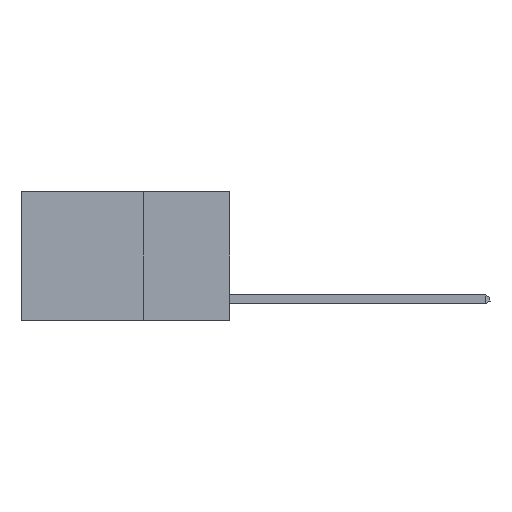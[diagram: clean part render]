
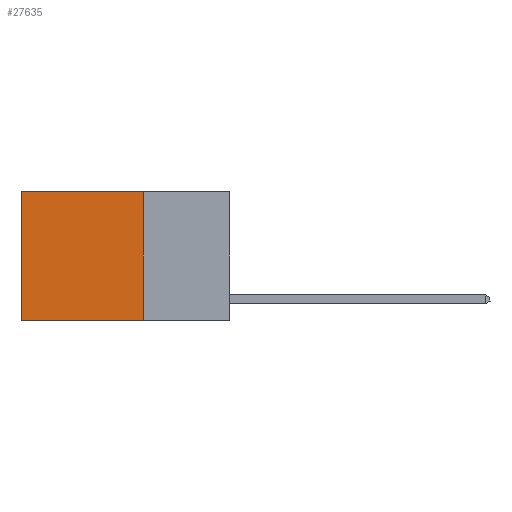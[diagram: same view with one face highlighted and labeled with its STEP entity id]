
A CAD part, left-side view. The second image highlights one B-rep face of the part: STEP entity #27635.
In plain terms, the highlighted planar face has unit normal (-1, 0, 0).
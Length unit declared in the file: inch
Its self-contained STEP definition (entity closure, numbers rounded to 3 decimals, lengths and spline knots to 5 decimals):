
#2119 = ORIENTED_EDGE ( 'NONE', *, *, #8490, .T. ) ;
#3707 = CARTESIAN_POINT ( 'NONE',  ( 0.2625, 0.25, -0.37 ) ) ;
#5511 = LINE ( 'NONE', #29322, #12261 ) ;
#5602 = AXIS2_PLACEMENT_3D ( 'NONE', #17072, #10039, #26756 ) ;
#6097 = LINE ( 'NONE', #23149, #17379 ) ;
#6677 = VERTEX_POINT ( 'NONE', #13374 ) ;
#8291 = LINE ( 'NONE', #10303, #20652 ) ;
#8490 = EDGE_CURVE ( 'NONE', #20368, #9967, #23485, .T. ) ;
#8872 = CARTESIAN_POINT ( 'NONE',  ( 0.2625, 0.6, 0. ) ) ;
#8935 = ORIENTED_EDGE ( 'NONE', *, *, #17023, .F. ) ;
#8991 = CARTESIAN_POINT ( 'NONE',  ( 0.2625, 0.6, 0. ) ) ;
#9967 = VERTEX_POINT ( 'NONE', #22264 ) ;
#10039 = DIRECTION ( 'NONE',  ( 1., 0., 0. ) ) ;
#10198 = DIRECTION ( 'NONE',  ( 0., 1., 0. ) ) ;
#10303 = CARTESIAN_POINT ( 'NONE',  ( 0.2625, 0.25, -0.37 ) ) ;
#11815 = VECTOR ( 'NONE', #28025, 39.37008 ) ;
#12261 = VECTOR ( 'NONE', #12357, 39.37008 ) ;
#12357 = DIRECTION ( 'NONE',  ( 0., 0., -1. ) ) ;
#13374 = CARTESIAN_POINT ( 'NONE',  ( 0.2625, 0.25, 0. ) ) ;
#13723 = ORIENTED_EDGE ( 'NONE', *, *, #22819, .T. ) ;
#16827 = EDGE_LOOP ( 'NONE', ( #2119, #8935, #21894, #13723 ) ) ;
#17023 = EDGE_CURVE ( 'NONE', #28780, #9967, #8291, .T. ) ;
#17072 = CARTESIAN_POINT ( 'NONE',  ( 0.2625, 0.25, 0. ) ) ;
#17379 = VECTOR ( 'NONE', #25351, 39.37008 ) ;
#20368 = VERTEX_POINT ( 'NONE', #8991 ) ;
#20652 = VECTOR ( 'NONE', #10198, 39.37008 ) ;
#21894 = ORIENTED_EDGE ( 'NONE', *, *, #26470, .F. ) ;
#22264 = CARTESIAN_POINT ( 'NONE',  ( 0.2625, 0.6, -0.37 ) ) ;
#22819 = EDGE_CURVE ( 'NONE', #6677, #20368, #6097, .T. ) ;
#23149 = CARTESIAN_POINT ( 'NONE',  ( 0.2625, 0.25, 0. ) ) ;
#23485 = LINE ( 'NONE', #8872, #11815 ) ;
#25351 = DIRECTION ( 'NONE',  ( 0., 1., 0. ) ) ;
#25763 = FACE_OUTER_BOUND ( 'NONE', #16827, .T. ) ;
#26470 = EDGE_CURVE ( 'NONE', #6677, #28780, #5511, .T. ) ;
#26756 = DIRECTION ( 'NONE',  ( 0., 0., -1. ) ) ;
#27635 = ADVANCED_FACE ( 'NONE', ( #25763 ), #28968, .F. ) ;
#28025 = DIRECTION ( 'NONE',  ( 0., 0., -1. ) ) ;
#28780 = VERTEX_POINT ( 'NONE', #3707 ) ;
#28968 = PLANE ( 'NONE',  #5602 ) ;
#29322 = CARTESIAN_POINT ( 'NONE',  ( 0.2625, 0.25, 0. ) ) ;
